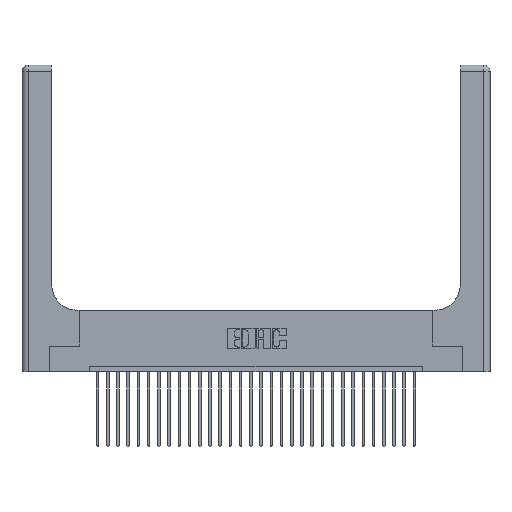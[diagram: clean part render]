
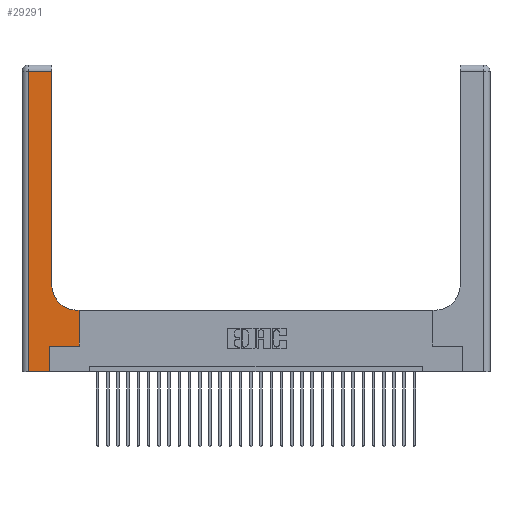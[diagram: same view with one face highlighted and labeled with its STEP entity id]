
A CAD part, top view. The second image highlights one B-rep face of the part: STEP entity #29291.
In plain terms, the highlighted planar face has unit normal (0, 0, 1).
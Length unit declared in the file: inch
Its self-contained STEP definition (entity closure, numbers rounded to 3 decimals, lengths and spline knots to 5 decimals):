
#255 = ORIENTED_EDGE ( 'NONE', *, *, #20307, .T. ) ;
#510 = ORIENTED_EDGE ( 'NONE', *, *, #7593, .T. ) ;
#733 = CIRCLE ( 'NONE', #13724, 0.25 ) ;
#1788 = AXIS2_PLACEMENT_3D ( 'NONE', #18409, #23179, #25860 ) ;
#1809 = DIRECTION ( 'NONE',  ( 1., 0., 0. ) ) ;
#2222 = ORIENTED_EDGE ( 'NONE', *, *, #19813, .T. ) ;
#3352 = VECTOR ( 'NONE', #7320, 39.37008 ) ;
#3555 = EDGE_CURVE ( 'NONE', #3987, #7190, #733, .T. ) ;
#3783 = VERTEX_POINT ( 'NONE', #5035 ) ;
#3868 = LINE ( 'NONE', #23010, #8332 ) ;
#3878 = CARTESIAN_POINT ( 'NONE',  ( 0.5585, 0.6, 0.37 ) ) ;
#3987 = VERTEX_POINT ( 'NONE', #27541 ) ;
#5035 = CARTESIAN_POINT ( 'NONE',  ( 0.06, 0., 0.37 ) ) ;
#5736 = CARTESIAN_POINT ( 'NONE',  ( 0.5415, 0.85, 0.37 ) ) ;
#5804 = DIRECTION ( 'NONE',  ( 1., 0., 0. ) ) ;
#5805 = VECTOR ( 'NONE', #19188, 39.37008 ) ;
#5996 = VERTEX_POINT ( 'NONE', #21027 ) ;
#6819 = VERTEX_POINT ( 'NONE', #3878 ) ;
#7008 = VERTEX_POINT ( 'NONE', #29994 ) ;
#7190 = VERTEX_POINT ( 'NONE', #15404 ) ;
#7221 = VERTEX_POINT ( 'NONE', #22398 ) ;
#7320 = DIRECTION ( 'NONE',  ( 0., 1., 0. ) ) ;
#7593 = EDGE_CURVE ( 'NONE', #27026, #6819, #13169, .T. ) ;
#7640 = VECTOR ( 'NONE', #16560, 39.37008 ) ;
#7793 = EDGE_CURVE ( 'NONE', #12557, #27026, #16496, .T. ) ;
#8332 = VECTOR ( 'NONE', #1809, 39.37008 ) ;
#8978 = VECTOR ( 'NONE', #26430, 39.37008 ) ;
#9693 = LINE ( 'NONE', #28013, #8978 ) ;
#10037 = CARTESIAN_POINT ( 'NONE',  ( 0.5585, 0.25, 0.37 ) ) ;
#10281 = ORIENTED_EDGE ( 'NONE', *, *, #20943, .T. ) ;
#10930 = VECTOR ( 'NONE', #25395, 39.37008 ) ;
#12085 = DIRECTION ( 'NONE',  ( 0., 0., -1. ) ) ;
#12557 = VERTEX_POINT ( 'NONE', #28919 ) ;
#12954 = LINE ( 'NONE', #28434, #3352 ) ;
#13169 = LINE ( 'NONE', #10037, #5805 ) ;
#13724 = AXIS2_PLACEMENT_3D ( 'NONE', #5736, #12085, #5804 ) ;
#14233 = CARTESIAN_POINT ( 'NONE',  ( 0.2915, 3., 0.37 ) ) ;
#14433 = DIRECTION ( 'NONE',  ( 0., 1., 0. ) ) ;
#14525 = VECTOR ( 'NONE', #14433, 39.37008 ) ;
#15404 = CARTESIAN_POINT ( 'NONE',  ( 0.2915, 0.85, 0.37 ) ) ;
#16123 = EDGE_CURVE ( 'NONE', #5996, #3783, #23812, .T. ) ;
#16260 = CARTESIAN_POINT ( 'NONE',  ( 0., 2.94, 0.37 ) ) ;
#16415 = ORIENTED_EDGE ( 'NONE', *, *, #30496, .T. ) ;
#16496 = LINE ( 'NONE', #20996, #10930 ) ;
#16560 = DIRECTION ( 'NONE',  ( -1., 0., 0. ) ) ;
#17231 = LINE ( 'NONE', #16260, #7640 ) ;
#18333 = EDGE_LOOP ( 'NONE', ( #2222, #16415, #25036, #24858, #10281, #28772, #510, #255, #19429 ) ) ;
#18409 = CARTESIAN_POINT ( 'NONE',  ( 0., 3., 0.37 ) ) ;
#18843 = FACE_OUTER_BOUND ( 'NONE', #18333, .T. ) ;
#19098 = EDGE_CURVE ( 'NONE', #3783, #7008, #3868, .T. ) ;
#19188 = DIRECTION ( 'NONE',  ( 0., 1., 0. ) ) ;
#19248 = DIRECTION ( 'NONE',  ( 0., -1., 0. ) ) ;
#19429 = ORIENTED_EDGE ( 'NONE', *, *, #3555, .T. ) ;
#19813 = EDGE_CURVE ( 'NONE', #7190, #7221, #26055, .T. ) ;
#20307 = EDGE_CURVE ( 'NONE', #6819, #3987, #9693, .T. ) ;
#20943 = EDGE_CURVE ( 'NONE', #7008, #12557, #12954, .T. ) ;
#20996 = CARTESIAN_POINT ( 'NONE',  ( 0.269, 0.25, 0.37 ) ) ;
#21027 = CARTESIAN_POINT ( 'NONE',  ( 0.06, 2.94, 0.37 ) ) ;
#22398 = CARTESIAN_POINT ( 'NONE',  ( 0.2915, 2.94, 0.37 ) ) ;
#23010 = CARTESIAN_POINT ( 'NONE',  ( 0., 0., 0.37 ) ) ;
#23179 = DIRECTION ( 'NONE',  ( 0., 0., -1. ) ) ;
#23812 = LINE ( 'NONE', #26792, #28655 ) ;
#24858 = ORIENTED_EDGE ( 'NONE', *, *, #19098, .T. ) ;
#25036 = ORIENTED_EDGE ( 'NONE', *, *, #16123, .T. ) ;
#25395 = DIRECTION ( 'NONE',  ( 1., 0., 0. ) ) ;
#25860 = DIRECTION ( 'NONE',  ( -1., 0., 0. ) ) ;
#25865 = CARTESIAN_POINT ( 'NONE',  ( 0.5585, 0.25, 0.37 ) ) ;
#26055 = LINE ( 'NONE', #14233, #14525 ) ;
#26430 = DIRECTION ( 'NONE',  ( -1., 0., 0. ) ) ;
#26792 = CARTESIAN_POINT ( 'NONE',  ( 0.06, 3., 0.37 ) ) ;
#27026 = VERTEX_POINT ( 'NONE', #25865 ) ;
#27541 = CARTESIAN_POINT ( 'NONE',  ( 0.5415, 0.6, 0.37 ) ) ;
#28013 = CARTESIAN_POINT ( 'NONE',  ( 0.2915, 0.6, 0.37 ) ) ;
#28434 = CARTESIAN_POINT ( 'NONE',  ( 0.269, 0., 0.37 ) ) ;
#28655 = VECTOR ( 'NONE', #19248, 39.37008 ) ;
#28772 = ORIENTED_EDGE ( 'NONE', *, *, #7793, .T. ) ;
#28919 = CARTESIAN_POINT ( 'NONE',  ( 0.269, 0.25, 0.37 ) ) ;
#29291 = ADVANCED_FACE ( 'NONE', ( #18843 ), #30135, .F. ) ;
#29994 = CARTESIAN_POINT ( 'NONE',  ( 0.269, 0., 0.37 ) ) ;
#30135 = PLANE ( 'NONE',  #1788 ) ;
#30496 = EDGE_CURVE ( 'NONE', #7221, #5996, #17231, .T. ) ;
